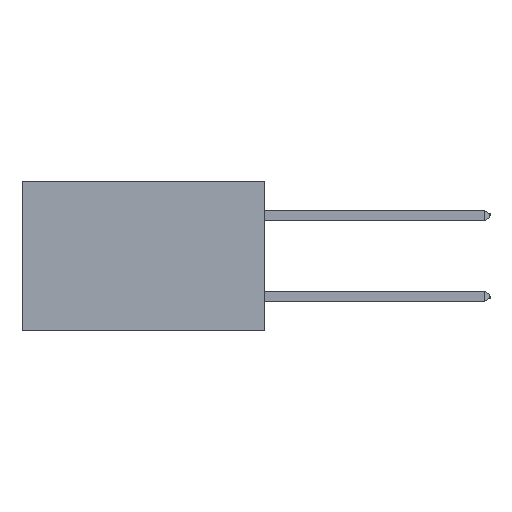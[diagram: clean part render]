
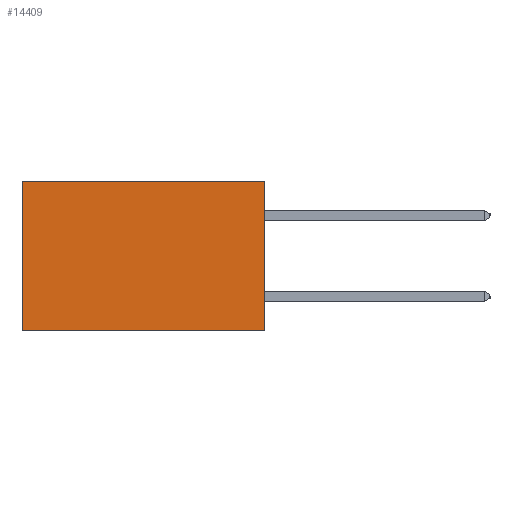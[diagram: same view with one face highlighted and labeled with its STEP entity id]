
A CAD part, left-side view. The second image highlights one B-rep face of the part: STEP entity #14409.
In plain terms, the highlighted planar face has unit normal (-1, 0, 0).
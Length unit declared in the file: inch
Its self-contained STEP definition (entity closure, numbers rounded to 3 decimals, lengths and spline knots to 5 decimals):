
#993 = VECTOR ( 'NONE', #13267, 39.37008 ) ;
#1914 = LINE ( 'NONE', #20497, #5872 ) ;
#3475 = CARTESIAN_POINT ( 'NONE',  ( 0.298, 0., 0. ) ) ;
#3981 = ORIENTED_EDGE ( 'NONE', *, *, #4958, .F. ) ;
#4408 = LINE ( 'NONE', #15619, #13063 ) ;
#4958 = EDGE_CURVE ( 'NONE', #19752, #9376, #12859, .T. ) ;
#5533 = CARTESIAN_POINT ( 'NONE',  ( 0.298, 0., 0. ) ) ;
#5872 = VECTOR ( 'NONE', #10729, 39.37008 ) ;
#6202 = DIRECTION ( 'NONE',  ( 0., 0., -1. ) ) ;
#6241 = CARTESIAN_POINT ( 'NONE',  ( 0.298, 0.6, -0.37 ) ) ;
#6280 = VERTEX_POINT ( 'NONE', #6241 ) ;
#7421 = DIRECTION ( 'NONE',  ( 1., 0., 0. ) ) ;
#8408 = CARTESIAN_POINT ( 'NONE',  ( 0.298, 0., 0. ) ) ;
#8587 = ORIENTED_EDGE ( 'NONE', *, *, #13275, .F. ) ;
#9124 = DIRECTION ( 'NONE',  ( 0., 0., -1. ) ) ;
#9376 = VERTEX_POINT ( 'NONE', #10945 ) ;
#10272 = EDGE_CURVE ( 'NONE', #19752, #13606, #14178, .T. ) ;
#10729 = DIRECTION ( 'NONE',  ( 0., 1., 0. ) ) ;
#10945 = CARTESIAN_POINT ( 'NONE',  ( 0.298, 0., -0.37 ) ) ;
#12619 = EDGE_LOOP ( 'NONE', ( #15450, #8587, #3981, #18396 ) ) ;
#12859 = LINE ( 'NONE', #5533, #18776 ) ;
#13063 = VECTOR ( 'NONE', #9124, 39.37008 ) ;
#13267 = DIRECTION ( 'NONE',  ( 0., 1., 0. ) ) ;
#13275 = EDGE_CURVE ( 'NONE', #9376, #6280, #1914, .T. ) ;
#13606 = VERTEX_POINT ( 'NONE', #14696 ) ;
#13894 = PLANE ( 'NONE',  #18564 ) ;
#14178 = LINE ( 'NONE', #3475, #993 ) ;
#14409 = ADVANCED_FACE ( 'NONE', ( #18546 ), #13894, .F. ) ;
#14696 = CARTESIAN_POINT ( 'NONE',  ( 0.298, 0.6, 0. ) ) ;
#15450 = ORIENTED_EDGE ( 'NONE', *, *, #18156, .T. ) ;
#15619 = CARTESIAN_POINT ( 'NONE',  ( 0.298, 0.6, 0. ) ) ;
#17186 = CARTESIAN_POINT ( 'NONE',  ( 0.298, 0., 0. ) ) ;
#18156 = EDGE_CURVE ( 'NONE', #13606, #6280, #4408, .T. ) ;
#18396 = ORIENTED_EDGE ( 'NONE', *, *, #10272, .T. ) ;
#18546 = FACE_OUTER_BOUND ( 'NONE', #12619, .T. ) ;
#18564 = AXIS2_PLACEMENT_3D ( 'NONE', #17186, #7421, #18834 ) ;
#18776 = VECTOR ( 'NONE', #6202, 39.37008 ) ;
#18834 = DIRECTION ( 'NONE',  ( 0., 0., -1. ) ) ;
#19752 = VERTEX_POINT ( 'NONE', #8408 ) ;
#20497 = CARTESIAN_POINT ( 'NONE',  ( 0.298, 0., -0.37 ) ) ;
